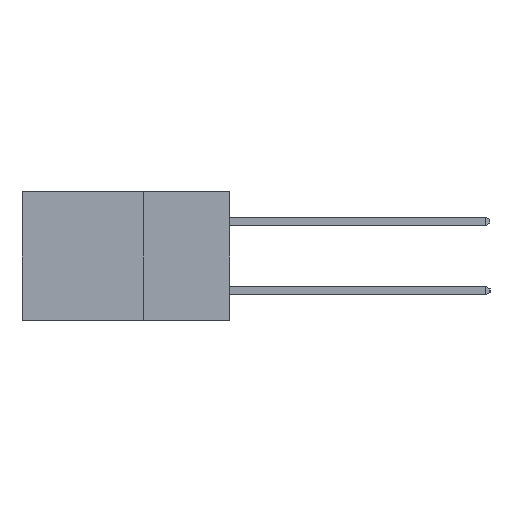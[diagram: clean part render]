
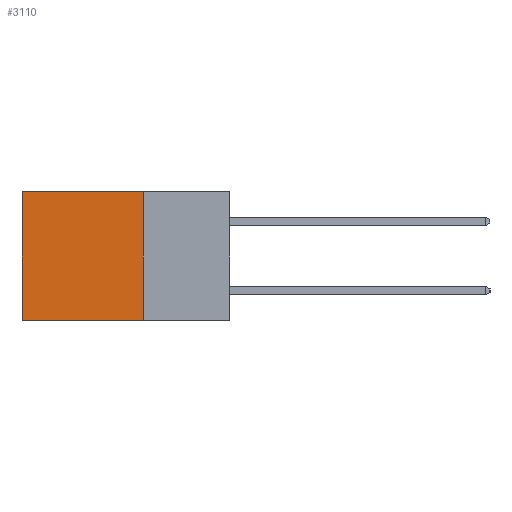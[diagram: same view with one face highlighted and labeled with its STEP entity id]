
A CAD part, left-side view. The second image highlights one B-rep face of the part: STEP entity #3110.
In plain terms, the highlighted planar face has unit normal (-1, 0, 0).
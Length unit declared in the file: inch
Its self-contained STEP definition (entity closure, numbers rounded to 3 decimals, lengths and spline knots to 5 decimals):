
#469 = AXIS2_PLACEMENT_3D ( 'NONE', #3122, #15234, #4882 ) ;
#498 = LINE ( 'NONE', #6119, #18557 ) ;
#1082 = VERTEX_POINT ( 'NONE', #8453 ) ;
#1265 = ORIENTED_EDGE ( 'NONE', *, *, #7306, .F. ) ;
#2193 = DIRECTION ( 'NONE',  ( 0., 1., 0. ) ) ;
#2525 = VECTOR ( 'NONE', #5173, 39.37008 ) ;
#2560 = DIRECTION ( 'NONE',  ( 0., 0., -1. ) ) ;
#3110 = ADVANCED_FACE ( 'NONE', ( #10773 ), #11786, .F. ) ;
#3122 = CARTESIAN_POINT ( 'NONE',  ( 0.2615, 0.25, -0.37 ) ) ;
#3380 = LINE ( 'NONE', #9558, #11526 ) ;
#4799 = EDGE_CURVE ( 'NONE', #6767, #10738, #19918, .T. ) ;
#4882 = DIRECTION ( 'NONE',  ( 0., 0., -1. ) ) ;
#4930 = EDGE_CURVE ( 'NONE', #1082, #20311, #3380, .T. ) ;
#5173 = DIRECTION ( 'NONE',  ( 0., 0., -1. ) ) ;
#5316 = CARTESIAN_POINT ( 'NONE',  ( 0.2615, 0.6, -0.37 ) ) ;
#5573 = VECTOR ( 'NONE', #2193, 39.37008 ) ;
#6119 = CARTESIAN_POINT ( 'NONE',  ( 0.2615, 0.6, -0.37 ) ) ;
#6767 = VERTEX_POINT ( 'NONE', #19223 ) ;
#7306 = EDGE_CURVE ( 'NONE', #1082, #6767, #12231, .T. ) ;
#7889 = DIRECTION ( 'NONE',  ( 0., 1., 0. ) ) ;
#8453 = CARTESIAN_POINT ( 'NONE',  ( 0.2615, 0.25, 0. ) ) ;
#9259 = CARTESIAN_POINT ( 'NONE',  ( 0.2615, 0.25, -0.37 ) ) ;
#9558 = CARTESIAN_POINT ( 'NONE',  ( 0.2615, 0.25, 0. ) ) ;
#10738 = VERTEX_POINT ( 'NONE', #5316 ) ;
#10773 = FACE_OUTER_BOUND ( 'NONE', #12753, .T. ) ;
#11526 = VECTOR ( 'NONE', #7889, 39.37008 ) ;
#11786 = PLANE ( 'NONE',  #469 ) ;
#12231 = LINE ( 'NONE', #13810, #2525 ) ;
#12753 = EDGE_LOOP ( 'NONE', ( #15651, #17010, #1265, #15419 ) ) ;
#13434 = EDGE_CURVE ( 'NONE', #20311, #10738, #498, .T. ) ;
#13771 = CARTESIAN_POINT ( 'NONE',  ( 0.2615, 0.6, 0. ) ) ;
#13810 = CARTESIAN_POINT ( 'NONE',  ( 0.2615, 0.25, -0.37 ) ) ;
#15234 = DIRECTION ( 'NONE',  ( 1., 0., 0. ) ) ;
#15419 = ORIENTED_EDGE ( 'NONE', *, *, #4930, .T. ) ;
#15651 = ORIENTED_EDGE ( 'NONE', *, *, #13434, .T. ) ;
#17010 = ORIENTED_EDGE ( 'NONE', *, *, #4799, .F. ) ;
#18557 = VECTOR ( 'NONE', #2560, 39.37008 ) ;
#19223 = CARTESIAN_POINT ( 'NONE',  ( 0.2615, 0.25, -0.37 ) ) ;
#19918 = LINE ( 'NONE', #9259, #5573 ) ;
#20311 = VERTEX_POINT ( 'NONE', #13771 ) ;
